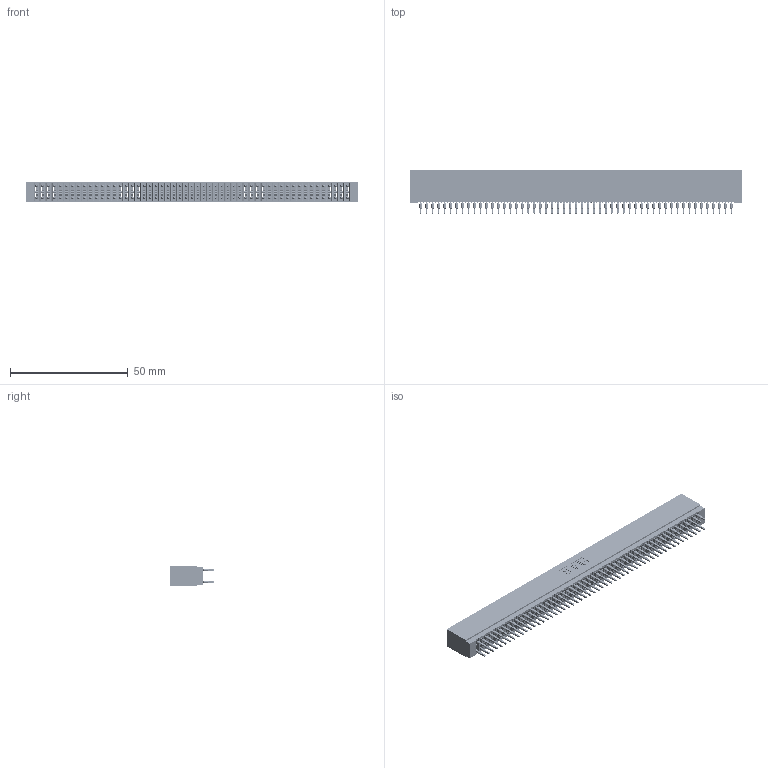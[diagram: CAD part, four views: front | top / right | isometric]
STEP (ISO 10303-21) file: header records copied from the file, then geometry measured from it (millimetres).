
FILE_DESCRIPTION (( 'STEP AP203' ), '1' );
FILE_NAME ('725-106-560-201.STEP', '2026-02-24T20:19:15', ( '' ), ( '' ), 'SwSTEP 2.0', 'SolidWorks 2023', '' );
FILE_SCHEMA (( 'CONFIG_CONTROL_DESIGN' ));
Length unit declared in the file: millimetre
Products named in the file (3): 745-292-001_560; 725 Part_Insulator Option - 01; 725-106-560-201
Assembly tree (107 placements, depth 2):
  725-106-560-201
    725 Part_Insulator Option - 01
    745-292-001_560  x106
Bounding box: 141.22 x 18.8 x 8.89 mm (x, y, z)
Volume: 11535.4 mm3; surface area: 26270.8 mm2
Topology: 107 solids, 107 shells, 10536 faces, 28821 edges, 18294 vertices
Faces by surface type: plane 5461, cylinder 2319, bspline 2120, torus 636
Entity records: 88012 total; most frequent: CARTESIAN_POINT 15765, ORIENTED_EDGE 15222, DIRECTION 13295, EDGE_CURVE 7611, VECTOR 7103, LINE 7103, VERTEX_POINT 4854, AXIS2_PLACEMENT_3D 3096
